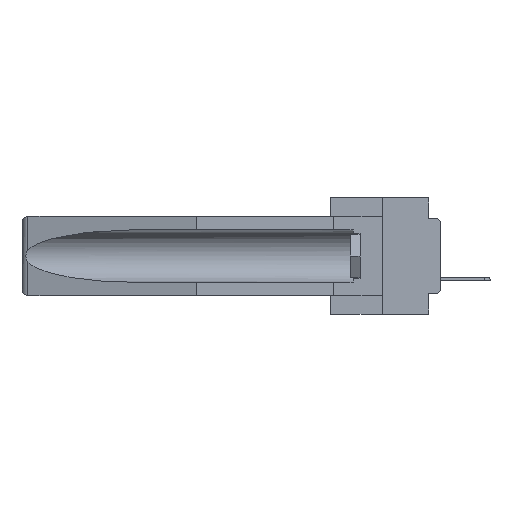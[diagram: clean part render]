
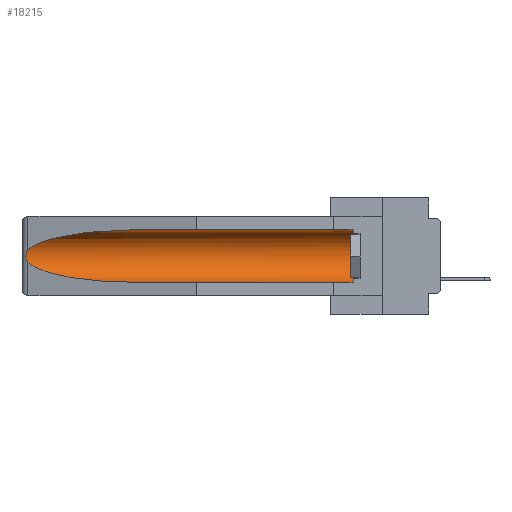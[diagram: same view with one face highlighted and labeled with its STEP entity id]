
A CAD part, left-side view. The second image highlights one B-rep face of the part: STEP entity #18215.
In plain terms, the highlighted cylindrical face has radius 2.857 mm (diameter 5.715 mm), a partial arc.
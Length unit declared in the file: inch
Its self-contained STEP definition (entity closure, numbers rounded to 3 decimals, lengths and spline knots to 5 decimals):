
#633 = CARTESIAN_POINT ( 'NONE',  ( 0.2673, 1.53269, -0.17917 ) ) ;
#780 = CARTESIAN_POINT ( 'NONE',  ( 0.26597, 1.5296, -0.19026 ) ) ;
#1835 = DIRECTION ( 'NONE',  ( 0., 1., 0. ) ) ;
#1888 = CYLINDRICAL_SURFACE ( 'NONE', #4157, 0.1125 ) ;
#2050 =( BOUNDED_CURVE ( )  B_SPLINE_CURVE ( 3, ( #23316, #12100, #11634, #2248 ),
 .UNSPECIFIED., .F., .F. ) 
 B_SPLINE_CURVE_WITH_KNOTS ( ( 4, 4 ),
 ( 4.71239, 6.08839 ),
 .UNSPECIFIED. ) 
 CURVE ( )  GEOMETRIC_REPRESENTATION_ITEM ( )  RATIONAL_B_SPLINE_CURVE ( ( 1., 0.848, 0.848, 1. ) ) 
 REPRESENTATION_ITEM ( '' )  );
#2248 = CARTESIAN_POINT ( 'NONE',  ( 0.26537, 1.52718, -0.14972 ) ) ;
#3126 = CARTESIAN_POINT ( 'NONE',  ( 0.155, 1.07973, -0.059 ) ) ;
#3395 = CARTESIAN_POINT ( 'NONE',  ( 0.26597, 1.52961, -0.15275 ) ) ;
#3951 = EDGE_CURVE ( 'NONE', #16134, #10203, #6404, .T. ) ;
#4157 = AXIS2_PLACEMENT_3D ( 'NONE', #11282, #20678, #30010 ) ;
#4291 = CARTESIAN_POINT ( 'NONE',  ( 0.155, 1.07973, -0.284 ) ) ;
#4402 = VERTEX_POINT ( 'NONE', #10552 ) ;
#5990 = LINE ( 'NONE', #10775, #20721 ) ;
#6404 = B_SPLINE_CURVE_WITH_KNOTS ( 'NONE', 3,
 ( #12486, #3395, #19582, #19426, #14936, #29067, #633, #10022, #780, #12794 ),
 .UNSPECIFIED., .F., .F.,
 ( 4, 2, 2, 2, 4 ),
 ( 0., 0.00029, 0.00058, 0.00087, 0.00117 ),
 .UNSPECIFIED. ) ;
#6444 = LINE ( 'NONE', #29951, #19675 ) ;
#6744 = ORIENTED_EDGE ( 'NONE', *, *, #15228, .T. ) ;
#7645 = CARTESIAN_POINT ( 'NONE',  ( 0.155, 0.126, -0.1715 ) ) ;
#7952 = DIRECTION ( 'NONE',  ( 0., -1., 0. ) ) ;
#9505 =( BOUNDED_CURVE ( )  B_SPLINE_CURVE ( 3, ( #14304, #29958, #14147, #4291 ),
 .UNSPECIFIED., .F., .F. ) 
 B_SPLINE_CURVE_WITH_KNOTS ( ( 4, 4 ),
 ( 0.1948, 1.5708 ),
 .UNSPECIFIED. ) 
 CURVE ( )  GEOMETRIC_REPRESENTATION_ITEM ( )  RATIONAL_B_SPLINE_CURVE ( ( 1., 0.848, 0.848, 1. ) ) 
 REPRESENTATION_ITEM ( '' )  );
#9923 = EDGE_CURVE ( 'NONE', #4402, #26339, #5990, .T. ) ;
#10022 = CARTESIAN_POINT ( 'NONE',  ( 0.26655, 1.53094, -0.18657 ) ) ;
#10060 = EDGE_CURVE ( 'NONE', #10203, #26339, #9505, .T. ) ;
#10203 = VERTEX_POINT ( 'NONE', #19537 ) ;
#10552 = CARTESIAN_POINT ( 'NONE',  ( 0.155, 0.126, -0.284 ) ) ;
#10775 = CARTESIAN_POINT ( 'NONE',  ( 0.155, -0.30754, -0.284 ) ) ;
#11282 = CARTESIAN_POINT ( 'NONE',  ( 0.155, -0.30754, -0.1715 ) ) ;
#11634 = CARTESIAN_POINT ( 'NONE',  ( 0.25451, 1.48313, -0.09465 ) ) ;
#12100 = CARTESIAN_POINT ( 'NONE',  ( 0.21114, 1.30732, -0.059 ) ) ;
#12436 = EDGE_CURVE ( 'NONE', #4402, #29271, #26619, .T. ) ;
#12486 = CARTESIAN_POINT ( 'NONE',  ( 0.26537, 1.52718, -0.14972 ) ) ;
#12794 = CARTESIAN_POINT ( 'NONE',  ( 0.26537, 1.52718, -0.19328 ) ) ;
#14147 = CARTESIAN_POINT ( 'NONE',  ( 0.21114, 1.30732, -0.284 ) ) ;
#14304 = CARTESIAN_POINT ( 'NONE',  ( 0.26537, 1.52718, -0.19328 ) ) ;
#14936 = CARTESIAN_POINT ( 'NONE',  ( 0.2675, 1.53308, -0.16763 ) ) ;
#15228 = EDGE_CURVE ( 'NONE', #16736, #16134, #2050, .T. ) ;
#16105 = ORIENTED_EDGE ( 'NONE', *, *, #12436, .T. ) ;
#16134 = VERTEX_POINT ( 'NONE', #19117 ) ;
#16736 = VERTEX_POINT ( 'NONE', #3126 ) ;
#16806 = ORIENTED_EDGE ( 'NONE', *, *, #3951, .T. ) ;
#17344 = DIRECTION ( 'NONE',  ( 0., 0., 1. ) ) ;
#18215 = ADVANCED_FACE ( 'NONE', ( #22967 ), #1888, .F. ) ;
#18490 = ORIENTED_EDGE ( 'NONE', *, *, #10060, .T. ) ;
#19117 = CARTESIAN_POINT ( 'NONE',  ( 0.26537, 1.52718, -0.14972 ) ) ;
#19426 = CARTESIAN_POINT ( 'NONE',  ( 0.2673, 1.5327, -0.16383 ) ) ;
#19537 = CARTESIAN_POINT ( 'NONE',  ( 0.26537, 1.52718, -0.19328 ) ) ;
#19582 = CARTESIAN_POINT ( 'NONE',  ( 0.26654, 1.53092, -0.15636 ) ) ;
#19675 = VECTOR ( 'NONE', #25972, 39.37008 ) ;
#20678 = DIRECTION ( 'NONE',  ( 0., 1., 0. ) ) ;
#20721 = VECTOR ( 'NONE', #1835, 39.37008 ) ;
#22967 = FACE_OUTER_BOUND ( 'NONE', #25481, .T. ) ;
#23316 = CARTESIAN_POINT ( 'NONE',  ( 0.155, 1.07973, -0.059 ) ) ;
#23414 = CARTESIAN_POINT ( 'NONE',  ( 0.155, 0.126, -0.059 ) ) ;
#24099 = ORIENTED_EDGE ( 'NONE', *, *, #9923, .F. ) ;
#24856 = ORIENTED_EDGE ( 'NONE', *, *, #24968, .T. ) ;
#24968 = EDGE_CURVE ( 'NONE', #29271, #16736, #6444, .T. ) ;
#25481 = EDGE_LOOP ( 'NONE', ( #6744, #16806, #18490, #24099, #16105, #24856 ) ) ;
#25972 = DIRECTION ( 'NONE',  ( 0., 1., 0. ) ) ;
#26339 = VERTEX_POINT ( 'NONE', #29682 ) ;
#26619 = CIRCLE ( 'NONE', #27570, 0.1125 ) ;
#27570 = AXIS2_PLACEMENT_3D ( 'NONE', #7645, #7952, #17344 ) ;
#29067 = CARTESIAN_POINT ( 'NONE',  ( 0.2675, 1.53308, -0.17534 ) ) ;
#29271 = VERTEX_POINT ( 'NONE', #23414 ) ;
#29682 = CARTESIAN_POINT ( 'NONE',  ( 0.155, 1.07973, -0.284 ) ) ;
#29951 = CARTESIAN_POINT ( 'NONE',  ( 0.155, -0.30754, -0.059 ) ) ;
#29958 = CARTESIAN_POINT ( 'NONE',  ( 0.25451, 1.48313, -0.24835 ) ) ;
#30010 = DIRECTION ( 'NONE',  ( 0., 0., 1. ) ) ;
